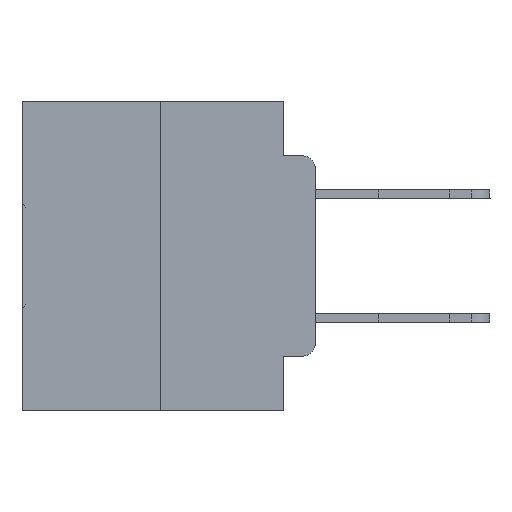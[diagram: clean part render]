
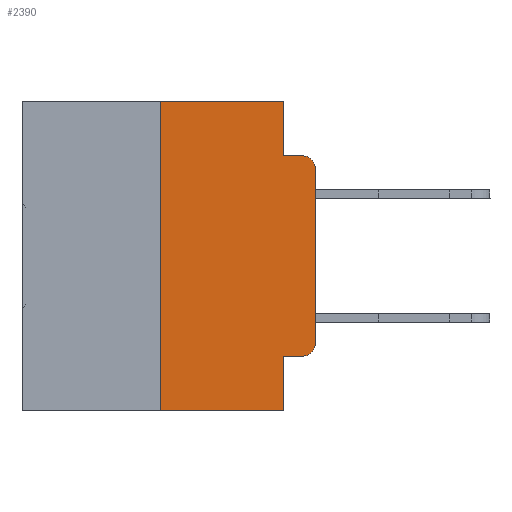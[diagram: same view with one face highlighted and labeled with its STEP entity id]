
A CAD part, left-side view. The second image highlights one B-rep face of the part: STEP entity #2390.
In plain terms, the highlighted planar face has unit normal (-1, 0, 0).
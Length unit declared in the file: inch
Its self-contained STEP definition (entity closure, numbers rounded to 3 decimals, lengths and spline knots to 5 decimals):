
#557 = VERTEX_POINT ( 'NONE', #26192 ) ;
#2327 = EDGE_CURVE ( 'NONE', #4867, #20090, #26071, .T. ) ;
#2390 = ADVANCED_FACE ( 'NONE', ( #11256 ), #20651, .F. ) ;
#3188 = DIRECTION ( 'NONE',  ( 0., 0., -1. ) ) ;
#3927 = DIRECTION ( 'NONE',  ( 0., 0., 1. ) ) ;
#3955 = AXIS2_PLACEMENT_3D ( 'NONE', #14928, #32296, #17441 ) ;
#4551 = LINE ( 'NONE', #22607, #30304 ) ;
#4804 = ORIENTED_EDGE ( 'NONE', *, *, #20753, .F. ) ;
#4867 = VERTEX_POINT ( 'NONE', #11959 ) ;
#5429 = DIRECTION ( 'NONE',  ( 0., -1., 0. ) ) ;
#5618 = CARTESIAN_POINT ( 'NONE',  ( 0., 0.473, 0. ) ) ;
#5718 = CARTESIAN_POINT ( 'NONE',  ( 0., 0.02, -0.0885 ) ) ;
#5870 = LINE ( 'NONE', #16797, #25816 ) ;
#5966 = CARTESIAN_POINT ( 'NONE',  ( 0., 0.051, 0. ) ) ;
#6222 = VECTOR ( 'NONE', #8477, 39.37008 ) ;
#7285 = VERTEX_POINT ( 'NONE', #14347 ) ;
#7387 = EDGE_CURVE ( 'NONE', #7285, #4867, #10662, .T. ) ;
#7955 = ORIENTED_EDGE ( 'NONE', *, *, #9025, .F. ) ;
#8477 = DIRECTION ( 'NONE',  ( 0., 0., -1. ) ) ;
#9025 = EDGE_CURVE ( 'NONE', #7285, #19158, #26149, .T. ) ;
#9050 = VECTOR ( 'NONE', #26727, 39.37008 ) ;
#9507 = CIRCLE ( 'NONE', #3955, 0.02 ) ;
#9650 = DIRECTION ( 'NONE',  ( 0., 0., -1. ) ) ;
#9774 = CARTESIAN_POINT ( 'NONE',  ( 0., 0., -0.3915 ) ) ;
#9904 = ORIENTED_EDGE ( 'NONE', *, *, #25790, .T. ) ;
#9953 = DIRECTION ( 'NONE',  ( 1., 0., 0. ) ) ;
#10040 = DIRECTION ( 'NONE',  ( 0., -1., 0. ) ) ;
#10562 = LINE ( 'NONE', #24978, #17197 ) ;
#10662 = LINE ( 'NONE', #26829, #9050 ) ;
#11256 = FACE_OUTER_BOUND ( 'NONE', #29695, .T. ) ;
#11959 = CARTESIAN_POINT ( 'NONE',  ( 0., 0.02, -0.4115 ) ) ;
#12296 = VERTEX_POINT ( 'NONE', #17510 ) ;
#12307 = AXIS2_PLACEMENT_3D ( 'NONE', #32223, #26282, #3188 ) ;
#12706 = DIRECTION ( 'NONE',  ( 0., 0., -1. ) ) ;
#13052 = ORIENTED_EDGE ( 'NONE', *, *, #14502, .T. ) ;
#13350 = CARTESIAN_POINT ( 'NONE',  ( 0., 0.051, 0. ) ) ;
#14099 = EDGE_CURVE ( 'NONE', #16287, #31025, #15623, .T. ) ;
#14234 = VECTOR ( 'NONE', #21520, 39.37008 ) ;
#14347 = CARTESIAN_POINT ( 'NONE',  ( 0., 0.051, -0.4115 ) ) ;
#14502 = EDGE_CURVE ( 'NONE', #16287, #19158, #22197, .T. ) ;
#14928 = CARTESIAN_POINT ( 'NONE',  ( 0., 0.02, -0.1085 ) ) ;
#15623 = LINE ( 'NONE', #21397, #27302 ) ;
#15697 = CARTESIAN_POINT ( 'NONE',  ( 0., 0.25, 0. ) ) ;
#16287 = VERTEX_POINT ( 'NONE', #30186 ) ;
#16797 = CARTESIAN_POINT ( 'NONE',  ( 0., 0., 0. ) ) ;
#17060 = VERTEX_POINT ( 'NONE', #13350 ) ;
#17197 = VECTOR ( 'NONE', #10040, 39.37008 ) ;
#17441 = DIRECTION ( 'NONE',  ( 0., 0., -1. ) ) ;
#17510 = CARTESIAN_POINT ( 'NONE',  ( 0., 0.051, -0.0885 ) ) ;
#18005 = CARTESIAN_POINT ( 'NONE',  ( 0., 0.473, -0.5 ) ) ;
#19030 = CARTESIAN_POINT ( 'NONE',  ( 0., 0.051, -0.0885 ) ) ;
#19158 = VERTEX_POINT ( 'NONE', #26722 ) ;
#19306 = DIRECTION ( 'NONE',  ( 0., 0., 1. ) ) ;
#20090 = VERTEX_POINT ( 'NONE', #9774 ) ;
#20651 = PLANE ( 'NONE',  #30651 ) ;
#20753 = EDGE_CURVE ( 'NONE', #17060, #12296, #4551, .T. ) ;
#21397 = CARTESIAN_POINT ( 'NONE',  ( 0., 0.25, 0. ) ) ;
#21426 = VECTOR ( 'NONE', #5429, 39.37008 ) ;
#21520 = DIRECTION ( 'NONE',  ( 0., -1., 0. ) ) ;
#22197 = LINE ( 'NONE', #18005, #21426 ) ;
#22420 = EDGE_CURVE ( 'NONE', #12296, #27807, #27478, .T. ) ;
#22607 = CARTESIAN_POINT ( 'NONE',  ( 0., 0.051, 0. ) ) ;
#23169 = ORIENTED_EDGE ( 'NONE', *, *, #22420, .F. ) ;
#24742 = ORIENTED_EDGE ( 'NONE', *, *, #30847, .F. ) ;
#24978 = CARTESIAN_POINT ( 'NONE',  ( 0., 0.473, 0. ) ) ;
#25790 = EDGE_CURVE ( 'NONE', #557, #27807, #9507, .T. ) ;
#25816 = VECTOR ( 'NONE', #19306, 39.37008 ) ;
#26071 = CIRCLE ( 'NONE', #12307, 0.02 ) ;
#26149 = LINE ( 'NONE', #5966, #6222 ) ;
#26192 = CARTESIAN_POINT ( 'NONE',  ( 0., 0., -0.1085 ) ) ;
#26282 = DIRECTION ( 'NONE',  ( -1., 0., 0. ) ) ;
#26722 = CARTESIAN_POINT ( 'NONE',  ( 0., 0.051, -0.5 ) ) ;
#26727 = DIRECTION ( 'NONE',  ( 0., -1., 0. ) ) ;
#26829 = CARTESIAN_POINT ( 'NONE',  ( 0., 0.051, -0.4115 ) ) ;
#27302 = VECTOR ( 'NONE', #3927, 39.37008 ) ;
#27434 = EDGE_CURVE ( 'NONE', #20090, #557, #5870, .T. ) ;
#27478 = LINE ( 'NONE', #19030, #14234 ) ;
#27807 = VERTEX_POINT ( 'NONE', #5718 ) ;
#27870 = ORIENTED_EDGE ( 'NONE', *, *, #7387, .T. ) ;
#28238 = ORIENTED_EDGE ( 'NONE', *, *, #27434, .T. ) ;
#29695 = EDGE_LOOP ( 'NONE', ( #28238, #9904, #23169, #4804, #24742, #31314, #13052, #7955, #27870, #30185 ) ) ;
#30185 = ORIENTED_EDGE ( 'NONE', *, *, #2327, .T. ) ;
#30186 = CARTESIAN_POINT ( 'NONE',  ( 0., 0.25, -0.5 ) ) ;
#30304 = VECTOR ( 'NONE', #12706, 39.37008 ) ;
#30651 = AXIS2_PLACEMENT_3D ( 'NONE', #5618, #9953, #9650 ) ;
#30847 = EDGE_CURVE ( 'NONE', #31025, #17060, #10562, .T. ) ;
#31025 = VERTEX_POINT ( 'NONE', #15697 ) ;
#31314 = ORIENTED_EDGE ( 'NONE', *, *, #14099, .F. ) ;
#32223 = CARTESIAN_POINT ( 'NONE',  ( 0., 0.02, -0.3915 ) ) ;
#32296 = DIRECTION ( 'NONE',  ( -1., 0., 0. ) ) ;
